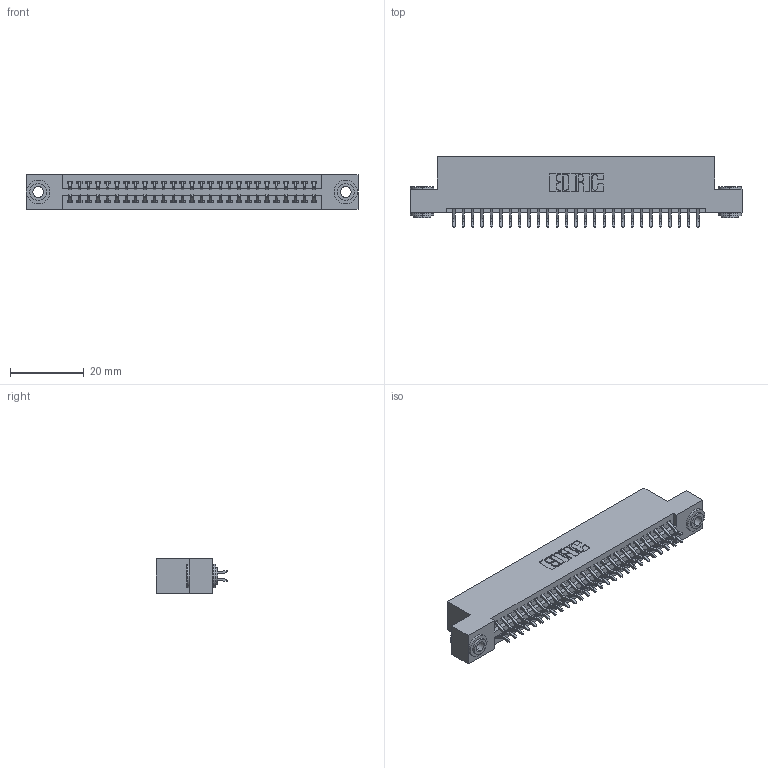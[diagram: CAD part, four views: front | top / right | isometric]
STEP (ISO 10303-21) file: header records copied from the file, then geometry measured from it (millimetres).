
FILE_DESCRIPTION (( 'STEP AP203' ), '1' );
FILE_NAME ('395-054-556-203.STEP', '2018-11-21T11:28:59', ( '' ), ( '' ), 'SwSTEP 2.0', 'SolidWorks 2016', '' );
FILE_SCHEMA (( 'CONFIG_CONTROL_DESIGN' ));
Length unit declared in the file: inch
Products named in the file (4): 395-054-556-203; 345 Part_Flush Mounting Lugs - 0.156 Dia-TH; 345-292-001_556 Tail; 345-250-002_345-250-002-102
Assembly tree (57 placements, depth 2):
  395-054-556-203
    345 Part_Flush Mounting Lugs - 0.156 Dia-TH
    345-292-001_556 Tail  x54
    345-250-002_345-250-002-102  x2
Bounding box: 89.79 x 19.24 x 9.4 mm (x, y, z)
Volume: 8600.2 mm3; surface area: 12579.7 mm2
Topology: 57 solids, 57 shells, 3188 faces, 9435 edges, 6214 vertices
Faces by surface type: plane 2088, cylinder 1092, cone 8
Entity records: 24074 total; most frequent: CARTESIAN_POINT 4039, ORIENTED_EDGE 3954, DIRECTION 3599, EDGE_CURVE 1977, VECTOR 1705, LINE 1705, VERTEX_POINT 1314, AXIS2_PLACEMENT_3D 947
